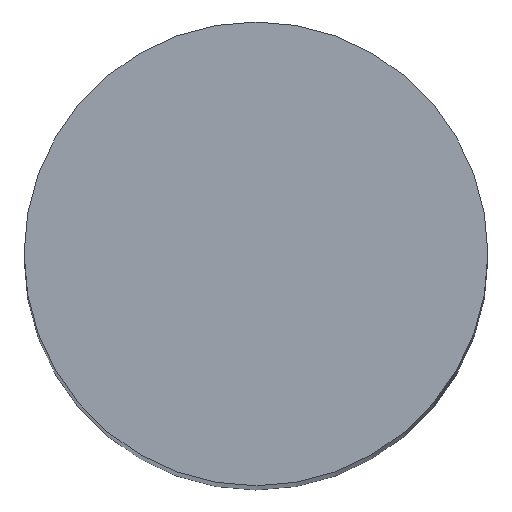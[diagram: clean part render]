
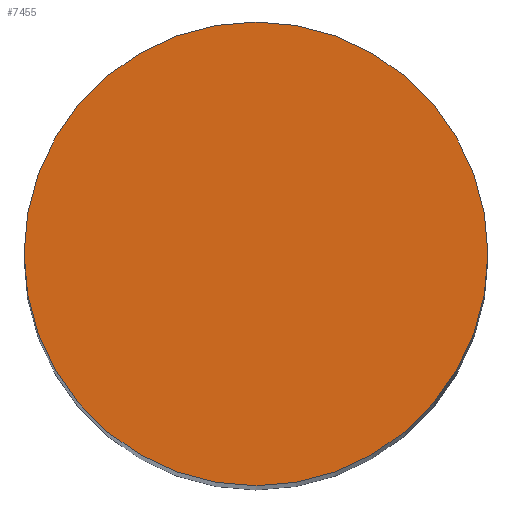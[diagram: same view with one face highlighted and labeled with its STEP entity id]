
A CAD part, top view. The second image highlights one B-rep face of the part: STEP entity #7455.
In plain terms, the highlighted planar face has unit normal (0, 0, 1).
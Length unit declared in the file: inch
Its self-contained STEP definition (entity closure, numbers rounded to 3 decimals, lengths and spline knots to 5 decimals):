
#649 = VERTEX_POINT ( 'NONE', #2804 ) ;
#1199 = DIRECTION ( 'NONE',  ( 0., 0., 1. ) ) ;
#1409 = EDGE_CURVE ( 'NONE', #649, #4166, #1726, .T. ) ;
#1726 = CIRCLE ( 'NONE', #7659, 0.645 ) ;
#2029 = CARTESIAN_POINT ( 'NONE',  ( -0.645, 0., -0.575 ) ) ;
#2263 = CARTESIAN_POINT ( 'NONE',  ( 0., 0., -0.575 ) ) ;
#2294 = PLANE ( 'NONE',  #7855 ) ;
#2609 = EDGE_LOOP ( 'NONE', ( #7206, #6556 ) ) ;
#2804 = CARTESIAN_POINT ( 'NONE',  ( 0.645, 0., -0.575 ) ) ;
#2822 = DIRECTION ( 'NONE',  ( 1., 0., 0. ) ) ;
#2860 = CARTESIAN_POINT ( 'NONE',  ( 0., 0., -0.575 ) ) ;
#2948 = DIRECTION ( 'NONE',  ( 0., 0., 1. ) ) ;
#3554 = DIRECTION ( 'NONE',  ( 0., 0., 1. ) ) ;
#4011 = CIRCLE ( 'NONE', #4260, 0.645 ) ;
#4166 = VERTEX_POINT ( 'NONE', #2029 ) ;
#4260 = AXIS2_PLACEMENT_3D ( 'NONE', #5068, #1199, #5710 ) ;
#5068 = CARTESIAN_POINT ( 'NONE',  ( 0., 0., -0.575 ) ) ;
#5710 = DIRECTION ( 'NONE',  ( 1., 0., 0. ) ) ;
#6556 = ORIENTED_EDGE ( 'NONE', *, *, #6830, .T. ) ;
#6830 = EDGE_CURVE ( 'NONE', #4166, #649, #4011, .T. ) ;
#7206 = ORIENTED_EDGE ( 'NONE', *, *, #1409, .T. ) ;
#7362 = DIRECTION ( 'NONE',  ( 1., 0., 0. ) ) ;
#7455 = ADVANCED_FACE ( 'NONE', ( #8010 ), #2294, .T. ) ;
#7659 = AXIS2_PLACEMENT_3D ( 'NONE', #2860, #3554, #2822 ) ;
#7855 = AXIS2_PLACEMENT_3D ( 'NONE', #2263, #2948, #7362 ) ;
#8010 = FACE_OUTER_BOUND ( 'NONE', #2609, .T. ) ;
